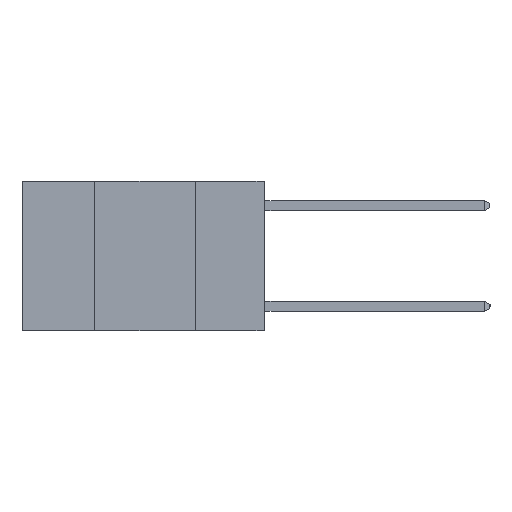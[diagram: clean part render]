
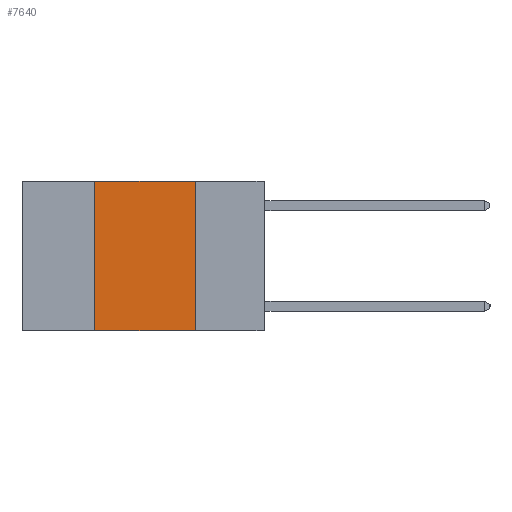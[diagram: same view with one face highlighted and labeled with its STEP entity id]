
A CAD part, left-side view. The second image highlights one B-rep face of the part: STEP entity #7640.
In plain terms, the highlighted planar face has unit normal (-1, 0, 0).
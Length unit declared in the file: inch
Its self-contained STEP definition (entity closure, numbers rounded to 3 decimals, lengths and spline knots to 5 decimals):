
#1 = VERTEX_POINT ( 'NONE', #2714 ) ;
#379 = ORIENTED_EDGE ( 'NONE', *, *, #1049, .T. ) ;
#531 = CARTESIAN_POINT ( 'NONE',  ( 0., 0.6, -0.37 ) ) ;
#903 = VECTOR ( 'NONE', #5034, 39.37008 ) ;
#1049 = EDGE_CURVE ( 'NONE', #5140, #9679, #9878, .T. ) ;
#1052 = EDGE_CURVE ( 'NONE', #5140, #1350, #7688, .T. ) ;
#1072 = EDGE_CURVE ( 'NONE', #1, #9679, #12081, .T. ) ;
#1143 = ORIENTED_EDGE ( 'NONE', *, *, #9408, .F. ) ;
#1336 = CARTESIAN_POINT ( 'NONE',  ( 0., 0.42, 0. ) ) ;
#1350 = VERTEX_POINT ( 'NONE', #1336 ) ;
#2283 = FACE_OUTER_BOUND ( 'NONE', #2871, .T. ) ;
#2361 = VECTOR ( 'NONE', #11122, 39.37008 ) ;
#2714 = CARTESIAN_POINT ( 'NONE',  ( 0., 0.17, 0. ) ) ;
#2871 = EDGE_LOOP ( 'NONE', ( #6169, #1143, #4903, #379 ) ) ;
#3606 = LINE ( 'NONE', #6799, #903 ) ;
#3639 = DIRECTION ( 'NONE',  ( 0., 0., -1. ) ) ;
#4600 = CARTESIAN_POINT ( 'NONE',  ( 0., 0.17, 0. ) ) ;
#4903 = ORIENTED_EDGE ( 'NONE', *, *, #1052, .F. ) ;
#5016 = VECTOR ( 'NONE', #10143, 39.37008 ) ;
#5034 = DIRECTION ( 'NONE',  ( 0., -1., 0. ) ) ;
#5140 = VERTEX_POINT ( 'NONE', #5484 ) ;
#5259 = AXIS2_PLACEMENT_3D ( 'NONE', #7498, #5734, #12184 ) ;
#5484 = CARTESIAN_POINT ( 'NONE',  ( 0., 0.42, -0.37 ) ) ;
#5579 = CARTESIAN_POINT ( 'NONE',  ( 0., 0.42, 0. ) ) ;
#5734 = DIRECTION ( 'NONE',  ( 1., 0., 0. ) ) ;
#6169 = ORIENTED_EDGE ( 'NONE', *, *, #1072, .F. ) ;
#6219 = CARTESIAN_POINT ( 'NONE',  ( 0., 0.17, -0.37 ) ) ;
#6799 = CARTESIAN_POINT ( 'NONE',  ( 0., 0.6, 0. ) ) ;
#7498 = CARTESIAN_POINT ( 'NONE',  ( 0., 0.6, 0. ) ) ;
#7640 = ADVANCED_FACE ( 'NONE', ( #2283 ), #11285, .F. ) ;
#7688 = LINE ( 'NONE', #5579, #5016 ) ;
#9308 = VECTOR ( 'NONE', #3639, 39.37008 ) ;
#9408 = EDGE_CURVE ( 'NONE', #1350, #1, #3606, .T. ) ;
#9679 = VERTEX_POINT ( 'NONE', #6219 ) ;
#9878 = LINE ( 'NONE', #531, #2361 ) ;
#10143 = DIRECTION ( 'NONE',  ( 0., 0., 1. ) ) ;
#11122 = DIRECTION ( 'NONE',  ( 0., -1., 0. ) ) ;
#11285 = PLANE ( 'NONE',  #5259 ) ;
#12081 = LINE ( 'NONE', #4600, #9308 ) ;
#12184 = DIRECTION ( 'NONE',  ( 0., 0., -1. ) ) ;
